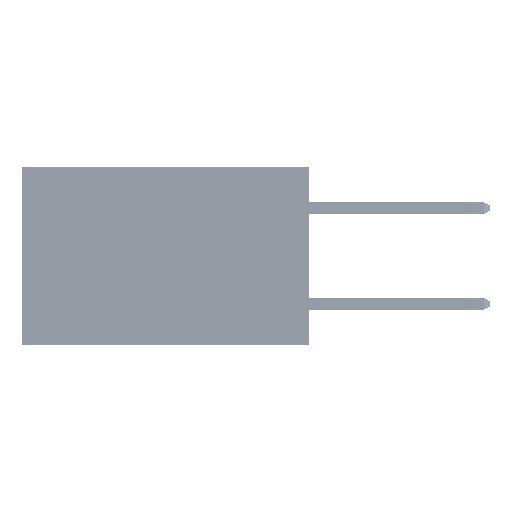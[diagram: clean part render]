
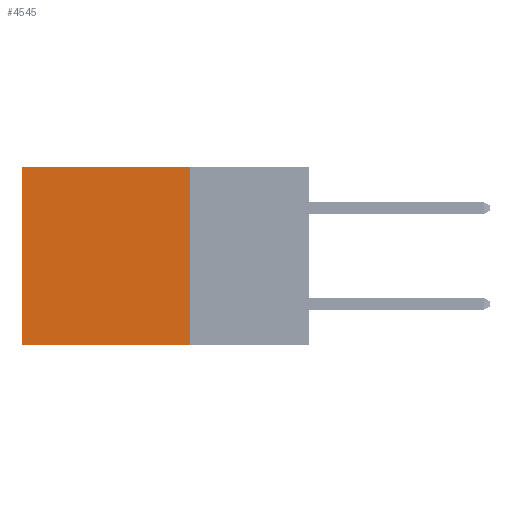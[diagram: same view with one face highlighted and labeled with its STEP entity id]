
A CAD part, left-side view. The second image highlights one B-rep face of the part: STEP entity #4545.
In plain terms, the highlighted planar face has unit normal (-1, 0, 0).
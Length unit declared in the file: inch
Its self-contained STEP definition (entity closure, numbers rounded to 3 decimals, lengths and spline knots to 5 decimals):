
#291 = VECTOR ( 'NONE', #35192, 39.37008 ) ;
#818 = LINE ( 'NONE', #43285, #37046 ) ;
#1690 = ORIENTED_EDGE ( 'NONE', *, *, #43311, .F. ) ;
#1732 = VERTEX_POINT ( 'NONE', #42500 ) ;
#4545 = ADVANCED_FACE ( 'NONE', ( #6576 ), #26127, .F. ) ;
#5159 = LINE ( 'NONE', #44530, #35427 ) ;
#6576 = FACE_OUTER_BOUND ( 'NONE', #15048, .T. ) ;
#6959 = DIRECTION ( 'NONE',  ( 0., 0., -1. ) ) ;
#7746 = ORIENTED_EDGE ( 'NONE', *, *, #14939, .F. ) ;
#9570 = LINE ( 'NONE', #35679, #47606 ) ;
#13242 = DIRECTION ( 'NONE',  ( 0., 0., -1. ) ) ;
#14792 = VERTEX_POINT ( 'NONE', #26599 ) ;
#14939 = EDGE_CURVE ( 'NONE', #33976, #14792, #9570, .T. ) ;
#15048 = EDGE_LOOP ( 'NONE', ( #44720, #1690, #7746, #47958 ) ) ;
#18510 = CARTESIAN_POINT ( 'NONE',  ( 0.2875, 0.25, 0. ) ) ;
#22469 = DIRECTION ( 'NONE',  ( 1., 0., 0. ) ) ;
#23665 = AXIS2_PLACEMENT_3D ( 'NONE', #18510, #22469, #37224 ) ;
#25249 = LINE ( 'NONE', #42383, #291 ) ;
#26127 = PLANE ( 'NONE',  #23665 ) ;
#26599 = CARTESIAN_POINT ( 'NONE',  ( 0.2875, 0.25, -0.37 ) ) ;
#30126 = EDGE_CURVE ( 'NONE', #33976, #47543, #818, .T. ) ;
#30775 = CARTESIAN_POINT ( 'NONE',  ( 0.2875, 0.25, 0. ) ) ;
#32285 = DIRECTION ( 'NONE',  ( 0., 1., 0. ) ) ;
#32574 = EDGE_CURVE ( 'NONE', #47543, #1732, #5159, .T. ) ;
#33976 = VERTEX_POINT ( 'NONE', #30775 ) ;
#35192 = DIRECTION ( 'NONE',  ( 0., 1., 0. ) ) ;
#35427 = VECTOR ( 'NONE', #6959, 39.37008 ) ;
#35679 = CARTESIAN_POINT ( 'NONE',  ( 0.2875, 0.25, 0. ) ) ;
#37046 = VECTOR ( 'NONE', #32285, 39.37008 ) ;
#37224 = DIRECTION ( 'NONE',  ( 0., 0., -1. ) ) ;
#42383 = CARTESIAN_POINT ( 'NONE',  ( 0.2875, 0.25, -0.37 ) ) ;
#42500 = CARTESIAN_POINT ( 'NONE',  ( 0.2875, 0.6, -0.37 ) ) ;
#43285 = CARTESIAN_POINT ( 'NONE',  ( 0.2875, 0.25, 0. ) ) ;
#43311 = EDGE_CURVE ( 'NONE', #14792, #1732, #25249, .T. ) ;
#44530 = CARTESIAN_POINT ( 'NONE',  ( 0.2875, 0.6, 0. ) ) ;
#44720 = ORIENTED_EDGE ( 'NONE', *, *, #32574, .T. ) ;
#47494 = CARTESIAN_POINT ( 'NONE',  ( 0.2875, 0.6, 0. ) ) ;
#47543 = VERTEX_POINT ( 'NONE', #47494 ) ;
#47606 = VECTOR ( 'NONE', #13242, 39.37008 ) ;
#47958 = ORIENTED_EDGE ( 'NONE', *, *, #30126, .T. ) ;
